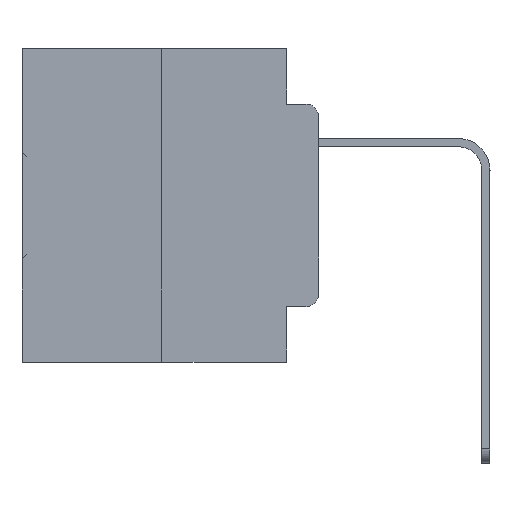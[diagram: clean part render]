
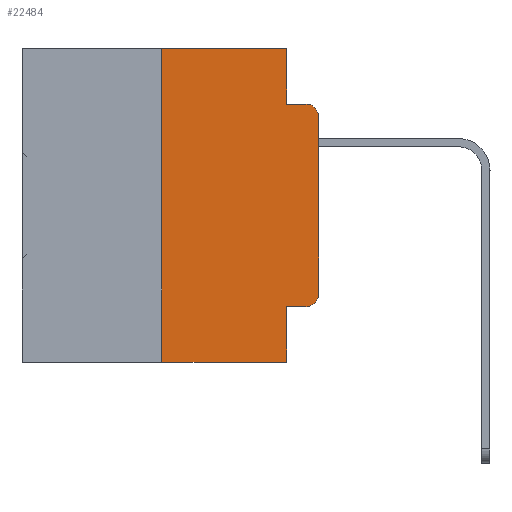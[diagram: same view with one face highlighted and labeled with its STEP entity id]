
A CAD part, left-side view. The second image highlights one B-rep face of the part: STEP entity #22484.
In plain terms, the highlighted planar face has unit normal (-1, 0, 0).
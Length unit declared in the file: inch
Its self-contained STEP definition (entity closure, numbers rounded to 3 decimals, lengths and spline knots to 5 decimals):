
#800 = EDGE_CURVE ( 'NONE', #34173, #28319, #6324, .T. ) ;
#1797 = VERTEX_POINT ( 'NONE', #28064 ) ;
#1844 = DIRECTION ( 'NONE',  ( 0., 0., 1. ) ) ;
#1874 = EDGE_LOOP ( 'NONE', ( #34289, #8974, #15309, #13316, #24400, #23151, #24294, #34251, #4624, #9921 ) ) ;
#2217 = VECTOR ( 'NONE', #29370, 39.37008 ) ;
#2509 = DIRECTION ( 'NONE',  ( 0., 0., -1. ) ) ;
#2914 = VERTEX_POINT ( 'NONE', #17492 ) ;
#3693 = EDGE_CURVE ( 'NONE', #1797, #22657, #21934, .T. ) ;
#4074 = CARTESIAN_POINT ( 'NONE',  ( 0., 0.02, -0.1085 ) ) ;
#4545 = VERTEX_POINT ( 'NONE', #19631 ) ;
#4624 = ORIENTED_EDGE ( 'NONE', *, *, #15375, .T. ) ;
#4776 = LINE ( 'NONE', #12949, #32112 ) ;
#6049 = CARTESIAN_POINT ( 'NONE',  ( 0., 0.02, -0.0885 ) ) ;
#6124 = CARTESIAN_POINT ( 'NONE',  ( 0., 0., -0.3915 ) ) ;
#6324 = CIRCLE ( 'NONE', #17113, 0.02 ) ;
#7123 = CARTESIAN_POINT ( 'NONE',  ( 0., 0.02, -0.4115 ) ) ;
#7157 = CIRCLE ( 'NONE', #17572, 0.02 ) ;
#7740 = DIRECTION ( 'NONE',  ( -1., 0., 0. ) ) ;
#8203 = DIRECTION ( 'NONE',  ( 1., 0., 0. ) ) ;
#8460 = VERTEX_POINT ( 'NONE', #25810 ) ;
#8463 = EDGE_CURVE ( 'NONE', #30556, #12011, #23899, .T. ) ;
#8974 = ORIENTED_EDGE ( 'NONE', *, *, #11523, .T. ) ;
#9827 = EDGE_CURVE ( 'NONE', #2914, #1797, #27125, .T. ) ;
#9921 = ORIENTED_EDGE ( 'NONE', *, *, #800, .T. ) ;
#10007 = VERTEX_POINT ( 'NONE', #21733 ) ;
#10492 = CARTESIAN_POINT ( 'NONE',  ( 0., 0.051, 0. ) ) ;
#10610 = VECTOR ( 'NONE', #33449, 39.37008 ) ;
#10627 = EDGE_CURVE ( 'NONE', #8460, #4545, #18339, .T. ) ;
#11523 = EDGE_CURVE ( 'NONE', #10007, #22657, #7157, .T. ) ;
#12011 = VERTEX_POINT ( 'NONE', #18412 ) ;
#12865 = CARTESIAN_POINT ( 'NONE',  ( 0., 0.051, -0.0885 ) ) ;
#12949 = CARTESIAN_POINT ( 'NONE',  ( 0., 0.051, -0.4115 ) ) ;
#13316 = ORIENTED_EDGE ( 'NONE', *, *, #9827, .F. ) ;
#14671 = CARTESIAN_POINT ( 'NONE',  ( 0., 0.473, 0. ) ) ;
#14711 = DIRECTION ( 'NONE',  ( 0., 0., -1. ) ) ;
#15309 = ORIENTED_EDGE ( 'NONE', *, *, #3693, .F. ) ;
#15375 = EDGE_CURVE ( 'NONE', #30556, #34173, #4776, .T. ) ;
#15500 = LINE ( 'NONE', #29259, #24637 ) ;
#16251 = DIRECTION ( 'NONE',  ( 0., -1., 0. ) ) ;
#17113 = AXIS2_PLACEMENT_3D ( 'NONE', #23608, #7740, #2509 ) ;
#17492 = CARTESIAN_POINT ( 'NONE',  ( 0., 0.051, 0. ) ) ;
#17572 = AXIS2_PLACEMENT_3D ( 'NONE', #4074, #22845, #14711 ) ;
#17657 = EDGE_CURVE ( 'NONE', #8460, #12011, #15500, .T. ) ;
#18252 = EDGE_CURVE ( 'NONE', #28319, #10007, #30389, .T. ) ;
#18339 = LINE ( 'NONE', #18690, #2217 ) ;
#18412 = CARTESIAN_POINT ( 'NONE',  ( 0., 0.051, -0.5 ) ) ;
#18690 = CARTESIAN_POINT ( 'NONE',  ( 0., 0.25, 0. ) ) ;
#19631 = CARTESIAN_POINT ( 'NONE',  ( 0., 0.25, 0. ) ) ;
#21660 = AXIS2_PLACEMENT_3D ( 'NONE', #23959, #8203, #29053 ) ;
#21733 = CARTESIAN_POINT ( 'NONE',  ( 0., 0., -0.1085 ) ) ;
#21934 = LINE ( 'NONE', #12865, #28962 ) ;
#22070 = LINE ( 'NONE', #14671, #27854 ) ;
#22165 = CARTESIAN_POINT ( 'NONE',  ( 0., 0.051, -0.4115 ) ) ;
#22484 = ADVANCED_FACE ( 'NONE', ( #23337 ), #32047, .F. ) ;
#22657 = VERTEX_POINT ( 'NONE', #6049 ) ;
#22845 = DIRECTION ( 'NONE',  ( -1., 0., 0. ) ) ;
#23019 = CARTESIAN_POINT ( 'NONE',  ( 0., 0.051, 0. ) ) ;
#23151 = ORIENTED_EDGE ( 'NONE', *, *, #10627, .F. ) ;
#23337 = FACE_OUTER_BOUND ( 'NONE', #1874, .T. ) ;
#23608 = CARTESIAN_POINT ( 'NONE',  ( 0., 0.02, -0.3915 ) ) ;
#23899 = LINE ( 'NONE', #23019, #10610 ) ;
#23959 = CARTESIAN_POINT ( 'NONE',  ( 0., 0.473, 0. ) ) ;
#24294 = ORIENTED_EDGE ( 'NONE', *, *, #17657, .T. ) ;
#24400 = ORIENTED_EDGE ( 'NONE', *, *, #31365, .F. ) ;
#24637 = VECTOR ( 'NONE', #16251, 39.37008 ) ;
#25810 = CARTESIAN_POINT ( 'NONE',  ( 0., 0.25, -0.5 ) ) ;
#27125 = LINE ( 'NONE', #10492, #32050 ) ;
#27511 = VECTOR ( 'NONE', #1844, 39.37008 ) ;
#27854 = VECTOR ( 'NONE', #28136, 39.37008 ) ;
#28064 = CARTESIAN_POINT ( 'NONE',  ( 0., 0.051, -0.0885 ) ) ;
#28136 = DIRECTION ( 'NONE',  ( 0., -1., 0. ) ) ;
#28147 = CARTESIAN_POINT ( 'NONE',  ( 0., 0., 0. ) ) ;
#28319 = VERTEX_POINT ( 'NONE', #6124 ) ;
#28962 = VECTOR ( 'NONE', #31422, 39.37008 ) ;
#29053 = DIRECTION ( 'NONE',  ( 0., 0., -1. ) ) ;
#29259 = CARTESIAN_POINT ( 'NONE',  ( 0., 0.473, -0.5 ) ) ;
#29357 = DIRECTION ( 'NONE',  ( 0., 0., -1. ) ) ;
#29370 = DIRECTION ( 'NONE',  ( 0., 0., 1. ) ) ;
#30389 = LINE ( 'NONE', #28147, #27511 ) ;
#30556 = VERTEX_POINT ( 'NONE', #22165 ) ;
#31365 = EDGE_CURVE ( 'NONE', #4545, #2914, #22070, .T. ) ;
#31422 = DIRECTION ( 'NONE',  ( 0., -1., 0. ) ) ;
#32047 = PLANE ( 'NONE',  #21660 ) ;
#32050 = VECTOR ( 'NONE', #29357, 39.37008 ) ;
#32112 = VECTOR ( 'NONE', #34186, 39.37008 ) ;
#33449 = DIRECTION ( 'NONE',  ( 0., 0., -1. ) ) ;
#34173 = VERTEX_POINT ( 'NONE', #7123 ) ;
#34186 = DIRECTION ( 'NONE',  ( 0., -1., 0. ) ) ;
#34251 = ORIENTED_EDGE ( 'NONE', *, *, #8463, .F. ) ;
#34289 = ORIENTED_EDGE ( 'NONE', *, *, #18252, .T. ) ;
